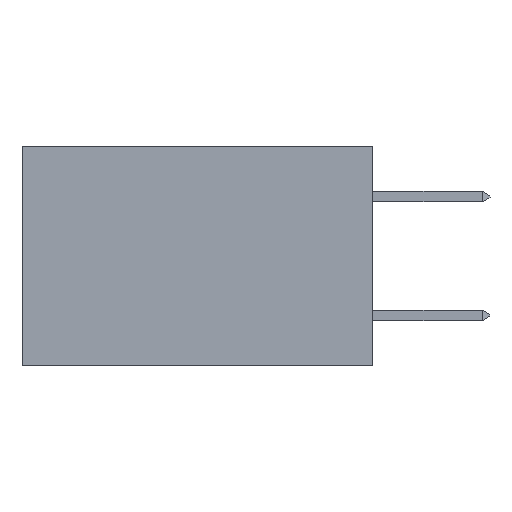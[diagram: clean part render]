
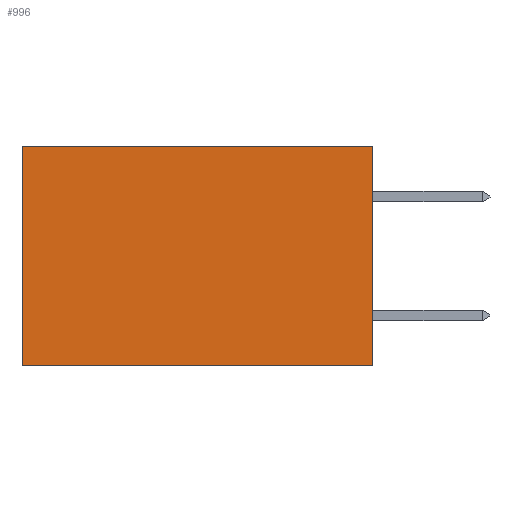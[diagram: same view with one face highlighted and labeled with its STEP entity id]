
A CAD part, left-side view. The second image highlights one B-rep face of the part: STEP entity #996.
In plain terms, the highlighted planar face has unit normal (-1, 0, 0).
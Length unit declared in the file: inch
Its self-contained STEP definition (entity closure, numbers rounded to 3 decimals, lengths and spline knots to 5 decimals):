
#85 = AXIS2_PLACEMENT_3D ( 'NONE', #9412, #3984, #3967 ) ;
#105 = ORIENTED_EDGE ( 'NONE', *, *, #175, .T. ) ;
#175 = EDGE_CURVE ( 'NONE', #4801, #4240, #8819, .T. ) ;
#277 = FACE_OUTER_BOUND ( 'NONE', #554, .T. ) ;
#554 = EDGE_LOOP ( 'NONE', ( #7387, #1673, #1343, #105 ) ) ;
#989 = VECTOR ( 'NONE', #3030, 39.37008 ) ;
#996 = ADVANCED_FACE ( 'NONE', ( #277 ), #4108, .F. ) ;
#1070 = LINE ( 'NONE', #5578, #6931 ) ;
#1343 = ORIENTED_EDGE ( 'NONE', *, *, #9709, .F. ) ;
#1673 = ORIENTED_EDGE ( 'NONE', *, *, #3481, .F. ) ;
#2281 = EDGE_CURVE ( 'NONE', #4240, #9135, #6448, .T. ) ;
#2325 = VERTEX_POINT ( 'NONE', #5271 ) ;
#2385 = VECTOR ( 'NONE', #8694, 39.37008 ) ;
#3030 = DIRECTION ( 'NONE',  ( 0., 1., 0. ) ) ;
#3481 = EDGE_CURVE ( 'NONE', #2325, #9135, #1070, .T. ) ;
#3967 = DIRECTION ( 'NONE',  ( 0., 0., -1. ) ) ;
#3984 = DIRECTION ( 'NONE',  ( 1., 0., 0. ) ) ;
#4108 = PLANE ( 'NONE',  #85 ) ;
#4240 = VERTEX_POINT ( 'NONE', #9150 ) ;
#4592 = VECTOR ( 'NONE', #7382, 39.37008 ) ;
#4801 = VERTEX_POINT ( 'NONE', #7193 ) ;
#5075 = LINE ( 'NONE', #5851, #4592 ) ;
#5271 = CARTESIAN_POINT ( 'NONE',  ( 0.277, 0., -0.37 ) ) ;
#5552 = DIRECTION ( 'NONE',  ( 0., 1., 0. ) ) ;
#5578 = CARTESIAN_POINT ( 'NONE',  ( 0.277, 0., -0.37 ) ) ;
#5851 = CARTESIAN_POINT ( 'NONE',  ( 0.277, 0., -0.37 ) ) ;
#6448 = LINE ( 'NONE', #9620, #2385 ) ;
#6931 = VECTOR ( 'NONE', #5552, 39.37008 ) ;
#7193 = CARTESIAN_POINT ( 'NONE',  ( 0.277, 0., 0. ) ) ;
#7382 = DIRECTION ( 'NONE',  ( 0., 0., -1. ) ) ;
#7387 = ORIENTED_EDGE ( 'NONE', *, *, #2281, .T. ) ;
#8190 = CARTESIAN_POINT ( 'NONE',  ( 0.277, 0.59, -0.37 ) ) ;
#8694 = DIRECTION ( 'NONE',  ( 0., 0., -1. ) ) ;
#8819 = LINE ( 'NONE', #9109, #989 ) ;
#9109 = CARTESIAN_POINT ( 'NONE',  ( 0.277, 0., 0. ) ) ;
#9135 = VERTEX_POINT ( 'NONE', #8190 ) ;
#9150 = CARTESIAN_POINT ( 'NONE',  ( 0.277, 0.59, 0. ) ) ;
#9412 = CARTESIAN_POINT ( 'NONE',  ( 0.277, 0., -0.37 ) ) ;
#9620 = CARTESIAN_POINT ( 'NONE',  ( 0.277, 0.59, -0.37 ) ) ;
#9709 = EDGE_CURVE ( 'NONE', #4801, #2325, #5075, .T. ) ;
